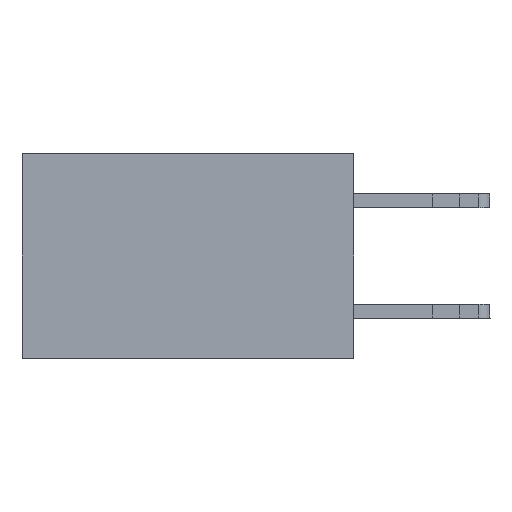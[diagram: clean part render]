
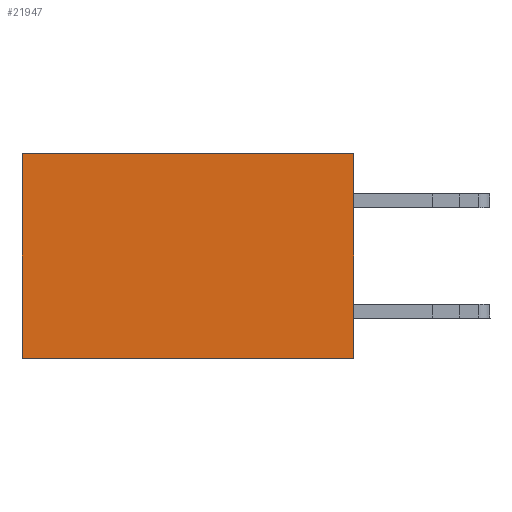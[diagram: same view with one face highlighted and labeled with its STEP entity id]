
A CAD part, left-side view. The second image highlights one B-rep face of the part: STEP entity #21947.
In plain terms, the highlighted planar face has unit normal (-1, 0, 0).
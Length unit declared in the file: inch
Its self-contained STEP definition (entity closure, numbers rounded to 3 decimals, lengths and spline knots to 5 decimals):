
#164 = ORIENTED_EDGE ( 'NONE', *, *, #25736, .F. ) ;
#2322 = VERTEX_POINT ( 'NONE', #23430 ) ;
#2433 = DIRECTION ( 'NONE',  ( 0., 1., 0. ) ) ;
#3446 = CARTESIAN_POINT ( 'NONE',  ( 0.2875, 0., 0. ) ) ;
#4485 = CARTESIAN_POINT ( 'NONE',  ( 0.2875, 0., -0.37 ) ) ;
#6378 = LINE ( 'NONE', #4485, #23353 ) ;
#6837 = VERTEX_POINT ( 'NONE', #26994 ) ;
#7381 = CARTESIAN_POINT ( 'NONE',  ( 0.2875, 0., 0. ) ) ;
#7432 = CARTESIAN_POINT ( 'NONE',  ( 0.2875, 0.6, -0.37 ) ) ;
#7443 = LINE ( 'NONE', #7381, #18998 ) ;
#7763 = ORIENTED_EDGE ( 'NONE', *, *, #27844, .T. ) ;
#8386 = FACE_OUTER_BOUND ( 'NONE', #9168, .T. ) ;
#9168 = EDGE_LOOP ( 'NONE', ( #7763, #24123, #164, #25896 ) ) ;
#9534 = DIRECTION ( 'NONE',  ( 0., 0., -1. ) ) ;
#10659 = DIRECTION ( 'NONE',  ( 0., 1., 0. ) ) ;
#12676 = DIRECTION ( 'NONE',  ( 0., 0., -1. ) ) ;
#15023 = VECTOR ( 'NONE', #9534, 39.37008 ) ;
#15835 = VERTEX_POINT ( 'NONE', #7432 ) ;
#17040 = CARTESIAN_POINT ( 'NONE',  ( 0.2875, 0.6, 0. ) ) ;
#17549 = EDGE_CURVE ( 'NONE', #18072, #2322, #28298, .T. ) ;
#18072 = VERTEX_POINT ( 'NONE', #3446 ) ;
#18998 = VECTOR ( 'NONE', #12676, 39.37008 ) ;
#19280 = CARTESIAN_POINT ( 'NONE',  ( 0.2875, 0., 0. ) ) ;
#19380 = PLANE ( 'NONE',  #20693 ) ;
#20693 = AXIS2_PLACEMENT_3D ( 'NONE', #19280, #29117, #21767 ) ;
#21767 = DIRECTION ( 'NONE',  ( 0., 0., -1. ) ) ;
#21947 = ADVANCED_FACE ( 'NONE', ( #8386 ), #19380, .F. ) ;
#22476 = EDGE_CURVE ( 'NONE', #6837, #15835, #6378, .T. ) ;
#23353 = VECTOR ( 'NONE', #2433, 39.37008 ) ;
#23430 = CARTESIAN_POINT ( 'NONE',  ( 0.2875, 0.6, 0. ) ) ;
#24123 = ORIENTED_EDGE ( 'NONE', *, *, #22476, .F. ) ;
#25736 = EDGE_CURVE ( 'NONE', #18072, #6837, #7443, .T. ) ;
#25896 = ORIENTED_EDGE ( 'NONE', *, *, #17549, .T. ) ;
#26994 = CARTESIAN_POINT ( 'NONE',  ( 0.2875, 0., -0.37 ) ) ;
#27844 = EDGE_CURVE ( 'NONE', #2322, #15835, #30852, .T. ) ;
#28298 = LINE ( 'NONE', #30580, #30969 ) ;
#29117 = DIRECTION ( 'NONE',  ( 1., 0., 0. ) ) ;
#30580 = CARTESIAN_POINT ( 'NONE',  ( 0.2875, 0., 0. ) ) ;
#30852 = LINE ( 'NONE', #17040, #15023 ) ;
#30969 = VECTOR ( 'NONE', #10659, 39.37008 ) ;
